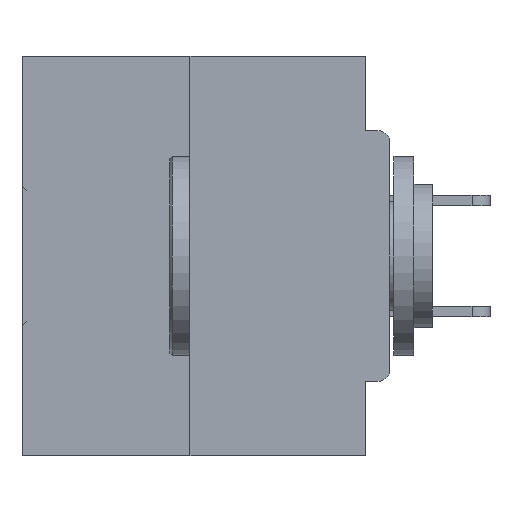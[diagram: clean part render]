
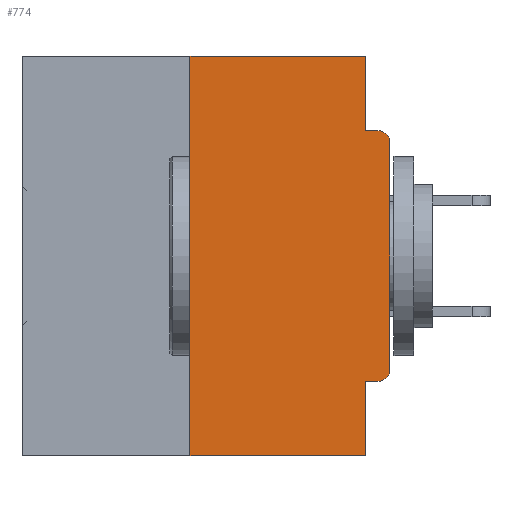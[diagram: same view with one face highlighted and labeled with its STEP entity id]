
A CAD part, left-side view. The second image highlights one B-rep face of the part: STEP entity #774.
In plain terms, the highlighted planar face has unit normal (-1, 0, 0).
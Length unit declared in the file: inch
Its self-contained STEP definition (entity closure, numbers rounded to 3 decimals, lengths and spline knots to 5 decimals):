
#774 = ADVANCED_FACE ( 'NONE', ( #25919 ), #24656, .F. ) ;
#1526 = ORIENTED_EDGE ( 'NONE', *, *, #2382, .T. ) ;
#1581 = ORIENTED_EDGE ( 'NONE', *, *, #12768, .T. ) ;
#2022 = ORIENTED_EDGE ( 'NONE', *, *, #34943, .T. ) ;
#2382 = EDGE_CURVE ( 'NONE', #33577, #24598, #39921, .T. ) ;
#3775 = VECTOR ( 'NONE', #28223, 39.37008 ) ;
#4315 = LINE ( 'NONE', #11300, #3775 ) ;
#4516 = DIRECTION ( 'NONE',  ( -1., 0., 0. ) ) ;
#4551 = ORIENTED_EDGE ( 'NONE', *, *, #34604, .T. ) ;
#4620 = VERTEX_POINT ( 'NONE', #10427 ) ;
#6281 = EDGE_CURVE ( 'NONE', #18738, #24598, #40155, .T. ) ;
#6625 = VECTOR ( 'NONE', #36581, 39.37008 ) ;
#6779 = CARTESIAN_POINT ( 'NONE',  ( 0., 0.015, -0.0935 ) ) ;
#7793 = CARTESIAN_POINT ( 'NONE',  ( 0., 0.015, -0.1085 ) ) ;
#7856 = CARTESIAN_POINT ( 'NONE',  ( 0., 0.015, -0.3915 ) ) ;
#8558 = EDGE_CURVE ( 'NONE', #29736, #4620, #15792, .T. ) ;
#8673 = CARTESIAN_POINT ( 'NONE',  ( 0., 0.031, -0.4065 ) ) ;
#9937 = EDGE_CURVE ( 'NONE', #10345, #29736, #25893, .T. ) ;
#10345 = VERTEX_POINT ( 'NONE', #31311 ) ;
#10358 = CARTESIAN_POINT ( 'NONE',  ( 0., 0.46, 0. ) ) ;
#10427 = CARTESIAN_POINT ( 'NONE',  ( 0., 0.031, -0.5 ) ) ;
#10529 = DIRECTION ( 'NONE',  ( 0., 0., -1. ) ) ;
#11250 = CARTESIAN_POINT ( 'NONE',  ( 0., 0.25, 0. ) ) ;
#11300 = CARTESIAN_POINT ( 'NONE',  ( 0., 0.031, 0. ) ) ;
#11661 = EDGE_CURVE ( 'NONE', #32142, #37324, #17706, .T. ) ;
#11759 = VERTEX_POINT ( 'NONE', #38221 ) ;
#12492 = LINE ( 'NONE', #24640, #24286 ) ;
#12768 = EDGE_CURVE ( 'NONE', #32142, #4620, #18671, .T. ) ;
#13368 = DIRECTION ( 'NONE',  ( 0., -1., 0. ) ) ;
#13564 = CIRCLE ( 'NONE', #37772, 0.015 ) ;
#14527 = ORIENTED_EDGE ( 'NONE', *, *, #11661, .F. ) ;
#14560 = DIRECTION ( 'NONE',  ( 0., 0., -1. ) ) ;
#15092 = DIRECTION ( 'NONE',  ( 0., 0., -1. ) ) ;
#15708 = DIRECTION ( 'NONE',  ( 0., 1., 0. ) ) ;
#15792 = LINE ( 'NONE', #29646, #6625 ) ;
#15842 = EDGE_CURVE ( 'NONE', #37324, #32463, #41462, .T. ) ;
#16771 = VECTOR ( 'NONE', #15708, 39.37008 ) ;
#16821 = DIRECTION ( 'NONE',  ( 0., -1., 0. ) ) ;
#17706 = LINE ( 'NONE', #11250, #43966 ) ;
#18114 = CARTESIAN_POINT ( 'NONE',  ( 0., 0.031, -0.0935 ) ) ;
#18671 = LINE ( 'NONE', #26443, #27707 ) ;
#18738 = VERTEX_POINT ( 'NONE', #18114 ) ;
#19587 = DIRECTION ( 'NONE',  ( 0., -1., 0. ) ) ;
#21527 = ORIENTED_EDGE ( 'NONE', *, *, #8558, .F. ) ;
#24286 = VECTOR ( 'NONE', #41564, 39.37008 ) ;
#24313 = CARTESIAN_POINT ( 'NONE',  ( 0., 0.25, 0. ) ) ;
#24519 = ORIENTED_EDGE ( 'NONE', *, *, #24652, .F. ) ;
#24598 = VERTEX_POINT ( 'NONE', #6779 ) ;
#24640 = CARTESIAN_POINT ( 'NONE',  ( 0., 0., 0. ) ) ;
#24652 = EDGE_CURVE ( 'NONE', #32463, #18738, #4315, .T. ) ;
#24656 = PLANE ( 'NONE',  #33757 ) ;
#24895 = CARTESIAN_POINT ( 'NONE',  ( 0., 0.031, 0. ) ) ;
#25211 = ORIENTED_EDGE ( 'NONE', *, *, #15842, .F. ) ;
#25666 = VECTOR ( 'NONE', #16821, 39.37008 ) ;
#25745 = CARTESIAN_POINT ( 'NONE',  ( 0., 0., -0.4065 ) ) ;
#25893 = LINE ( 'NONE', #25745, #16771 ) ;
#25919 = FACE_OUTER_BOUND ( 'NONE', #38845, .T. ) ;
#26443 = CARTESIAN_POINT ( 'NONE',  ( 0., 0.46, -0.5 ) ) ;
#27707 = VECTOR ( 'NONE', #19587, 39.37008 ) ;
#28204 = CARTESIAN_POINT ( 'NONE',  ( 0., 0., -0.1085 ) ) ;
#28223 = DIRECTION ( 'NONE',  ( 0., 0., -1. ) ) ;
#29646 = CARTESIAN_POINT ( 'NONE',  ( 0., 0.031, -0.5 ) ) ;
#29736 = VERTEX_POINT ( 'NONE', #8673 ) ;
#30940 = CARTESIAN_POINT ( 'NONE',  ( 0., 0.46, 0. ) ) ;
#31311 = CARTESIAN_POINT ( 'NONE',  ( 0., 0.015, -0.4065 ) ) ;
#32142 = VERTEX_POINT ( 'NONE', #43411 ) ;
#32390 = VECTOR ( 'NONE', #13368, 39.37008 ) ;
#32463 = VERTEX_POINT ( 'NONE', #24895 ) ;
#33577 = VERTEX_POINT ( 'NONE', #28204 ) ;
#33757 = AXIS2_PLACEMENT_3D ( 'NONE', #30940, #34408, #10529 ) ;
#34408 = DIRECTION ( 'NONE',  ( 1., 0., 0. ) ) ;
#34604 = EDGE_CURVE ( 'NONE', #10345, #11759, #13564, .T. ) ;
#34943 = EDGE_CURVE ( 'NONE', #11759, #33577, #12492, .T. ) ;
#35108 = DIRECTION ( 'NONE',  ( -1., 0., 0. ) ) ;
#35265 = DIRECTION ( 'NONE',  ( 0., 0., 1. ) ) ;
#36581 = DIRECTION ( 'NONE',  ( 0., 0., -1. ) ) ;
#37066 = CARTESIAN_POINT ( 'NONE',  ( 0., 0., -0.0935 ) ) ;
#37190 = ORIENTED_EDGE ( 'NONE', *, *, #6281, .F. ) ;
#37324 = VERTEX_POINT ( 'NONE', #24313 ) ;
#37772 = AXIS2_PLACEMENT_3D ( 'NONE', #7856, #4516, #15092 ) ;
#38221 = CARTESIAN_POINT ( 'NONE',  ( 0., 0., -0.3915 ) ) ;
#38446 = AXIS2_PLACEMENT_3D ( 'NONE', #7793, #35108, #14560 ) ;
#38673 = ORIENTED_EDGE ( 'NONE', *, *, #9937, .F. ) ;
#38845 = EDGE_LOOP ( 'NONE', ( #25211, #14527, #1581, #21527, #38673, #4551, #2022, #1526, #37190, #24519 ) ) ;
#39921 = CIRCLE ( 'NONE', #38446, 0.015 ) ;
#40155 = LINE ( 'NONE', #37066, #25666 ) ;
#41462 = LINE ( 'NONE', #10358, #32390 ) ;
#41564 = DIRECTION ( 'NONE',  ( 0., 0., 1. ) ) ;
#43411 = CARTESIAN_POINT ( 'NONE',  ( 0., 0.25, -0.5 ) ) ;
#43966 = VECTOR ( 'NONE', #35265, 39.37008 ) ;
